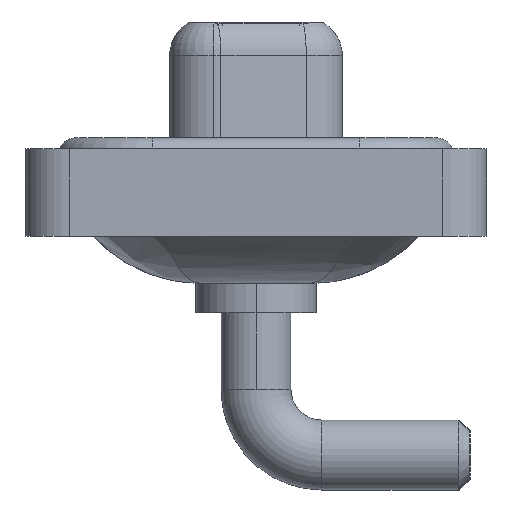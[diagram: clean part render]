
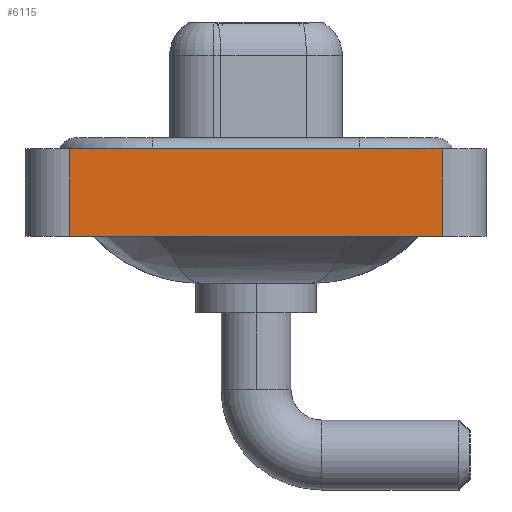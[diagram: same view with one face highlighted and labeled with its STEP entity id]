
A CAD part, left-side view. The second image highlights one B-rep face of the part: STEP entity #6115.
In plain terms, the highlighted planar face has unit normal (-1, 0, 0).
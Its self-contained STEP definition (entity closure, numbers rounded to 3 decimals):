
#274 = VERTEX_POINT ( 'NONE', #7264 ) ;
#309 = VECTOR ( 'NONE', #16495, 1000. ) ;
#1282 = EDGE_LOOP ( 'NONE', ( #5810, #15987, #11713, #3217 ) ) ;
#1512 = VERTEX_POINT ( 'NONE', #9444 ) ;
#1945 = CARTESIAN_POINT ( 'NONE',  ( -7.25, -8.55, -3.6 ) ) ;
#2135 = EDGE_CURVE ( 'NONE', #274, #3949, #14254, .T. ) ;
#3217 = ORIENTED_EDGE ( 'NONE', *, *, #2135, .T. ) ;
#3640 = AXIS2_PLACEMENT_3D ( 'NONE', #1945, #11790, #10905 ) ;
#3949 = VERTEX_POINT ( 'NONE', #16167 ) ;
#4513 = FACE_OUTER_BOUND ( 'NONE', #1282, .T. ) ;
#4521 = DIRECTION ( 'NONE',  ( 0., -1., 0. ) ) ;
#4691 = LINE ( 'NONE', #5965, #15731 ) ;
#5810 = ORIENTED_EDGE ( 'NONE', *, *, #5823, .T. ) ;
#5823 = EDGE_CURVE ( 'NONE', #3949, #1512, #12830, .T. ) ;
#5965 = CARTESIAN_POINT ( 'NONE',  ( -7.25, -8.55, 0.4 ) ) ;
#6104 = LINE ( 'NONE', #11320, #309 ) ;
#6115 = ADVANCED_FACE ( 'NONE', ( #4513 ), #10598, .T. ) ;
#7163 = EDGE_CURVE ( 'NONE', #274, #12318, #6104, .T. ) ;
#7264 = CARTESIAN_POINT ( 'NONE',  ( -7.25, 8.55, -3.6 ) ) ;
#7695 = VECTOR ( 'NONE', #15474, 1000. ) ;
#7758 = CARTESIAN_POINT ( 'NONE',  ( -7.25, 8.55, 0.4 ) ) ;
#9444 = CARTESIAN_POINT ( 'NONE',  ( -7.25, -8.55, 0.4 ) ) ;
#10110 = CARTESIAN_POINT ( 'NONE',  ( -7.25, -8.55, -3.6 ) ) ;
#10348 = CARTESIAN_POINT ( 'NONE',  ( -7.25, -8.55, -3.6 ) ) ;
#10592 = DIRECTION ( 'NONE',  ( 0., -1., 0. ) ) ;
#10598 = PLANE ( 'NONE',  #3640 ) ;
#10905 = DIRECTION ( 'NONE',  ( 0., 0., 1. ) ) ;
#11134 = VECTOR ( 'NONE', #10592, 1000. ) ;
#11320 = CARTESIAN_POINT ( 'NONE',  ( -7.25, 8.55, -3.6 ) ) ;
#11713 = ORIENTED_EDGE ( 'NONE', *, *, #7163, .F. ) ;
#11790 = DIRECTION ( 'NONE',  ( -1., 0., 0. ) ) ;
#12318 = VERTEX_POINT ( 'NONE', #7758 ) ;
#12830 = LINE ( 'NONE', #10110, #7695 ) ;
#14254 = LINE ( 'NONE', #10348, #11134 ) ;
#15474 = DIRECTION ( 'NONE',  ( 0., 0., 1. ) ) ;
#15667 = EDGE_CURVE ( 'NONE', #12318, #1512, #4691, .T. ) ;
#15731 = VECTOR ( 'NONE', #4521, 1000. ) ;
#15987 = ORIENTED_EDGE ( 'NONE', *, *, #15667, .F. ) ;
#16167 = CARTESIAN_POINT ( 'NONE',  ( -7.25, -8.55, -3.6 ) ) ;
#16495 = DIRECTION ( 'NONE',  ( 0., 0., 1. ) ) ;
